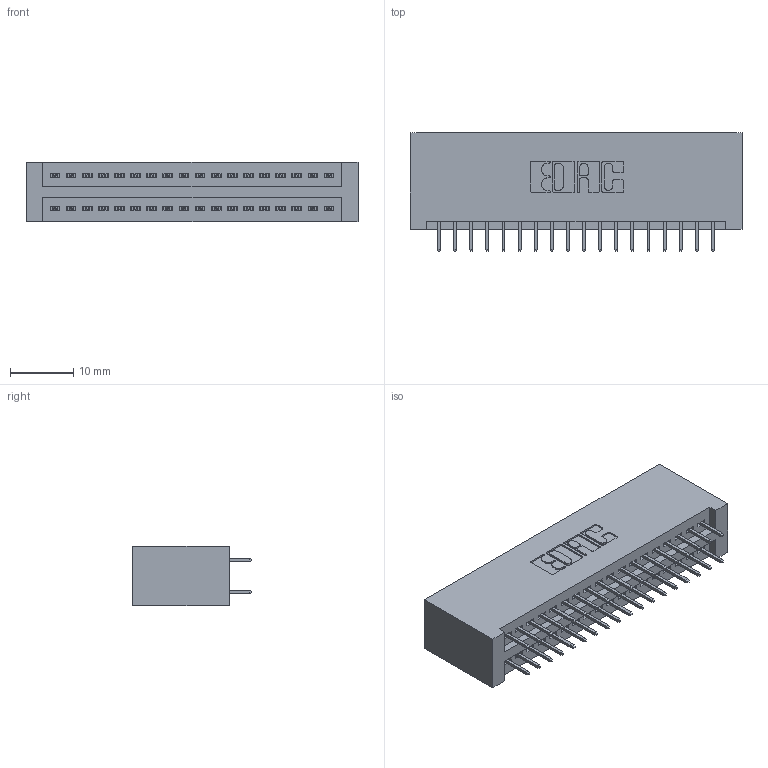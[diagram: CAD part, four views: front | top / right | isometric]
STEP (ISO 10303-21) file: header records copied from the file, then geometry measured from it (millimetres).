
FILE_DESCRIPTION (( 'STEP AP203' ), '1' );
FILE_NAME ('895-036-525-201.STEP', '2020-09-25T23:33:05', ( '' ), ( '' ), 'SwSTEP 2.0', 'SolidWorks 2020', '' );
FILE_SCHEMA (( 'CONFIG_CONTROL_DESIGN' ));
Length unit declared in the file: inch
Products named in the file (3): 845 Part_No Mounting Lugs; 895-036-525-201; 345-292-001_345-293-125
Assembly tree (37 placements, depth 2):
  895-036-525-201
    845 Part_No Mounting Lugs
    345-292-001_345-293-125  x36
Bounding box: 52.32 x 18.72 x 9.4 mm (x, y, z)
Volume: 5416.7 mm3; surface area: 7666.6 mm2
Topology: 37 solids, 37 shells, 2062 faces, 5825 edges, 3738 vertices
Faces by surface type: plane 1480, cylinder 582
Entity records: 17151 total; most frequent: CARTESIAN_POINT 2896, ORIENTED_EDGE 2830, DIRECTION 2579, EDGE_CURVE 1415, VECTOR 1223, LINE 1223, VERTEX_POINT 938, AXIS2_PLACEMENT_3D 678
